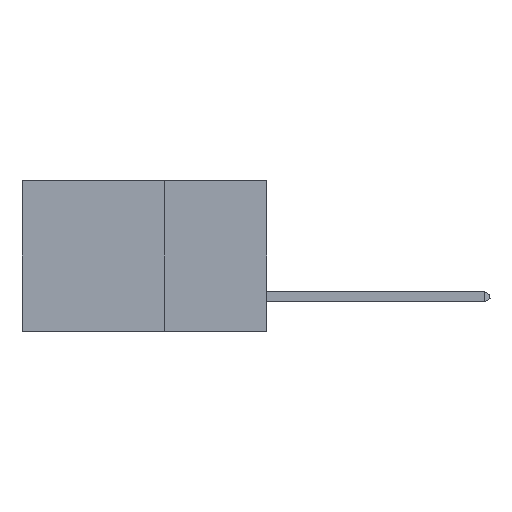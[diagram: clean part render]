
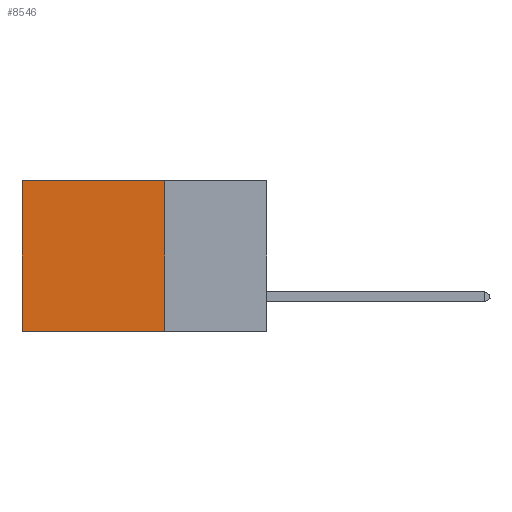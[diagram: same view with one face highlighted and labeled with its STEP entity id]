
A CAD part, left-side view. The second image highlights one B-rep face of the part: STEP entity #8546.
In plain terms, the highlighted planar face has unit normal (-1, 0, 0).
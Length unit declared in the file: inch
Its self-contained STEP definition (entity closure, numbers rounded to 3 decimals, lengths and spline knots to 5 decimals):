
#838 = DIRECTION ( 'NONE',  ( 0., 1., 0. ) ) ;
#1077 = CARTESIAN_POINT ( 'NONE',  ( 0.2875, 0.25, -0.37 ) ) ;
#1241 = EDGE_LOOP ( 'NONE', ( #8976, #8566, #4167, #13422 ) ) ;
#1479 = VECTOR ( 'NONE', #16630, 39.37008 ) ;
#1758 = VERTEX_POINT ( 'NONE', #14915 ) ;
#1759 = CARTESIAN_POINT ( 'NONE',  ( 0.2875, 0.6, 0. ) ) ;
#2491 = LINE ( 'NONE', #5364, #2725 ) ;
#2725 = VECTOR ( 'NONE', #15488, 39.37008 ) ;
#2835 = PLANE ( 'NONE',  #13558 ) ;
#3057 = VERTEX_POINT ( 'NONE', #8640 ) ;
#3827 = CARTESIAN_POINT ( 'NONE',  ( 0.2875, 0.25, -0.37 ) ) ;
#4167 = ORIENTED_EDGE ( 'NONE', *, *, #18535, .F. ) ;
#4817 = VERTEX_POINT ( 'NONE', #9337 ) ;
#5364 = CARTESIAN_POINT ( 'NONE',  ( 0.2875, 0.25, 0. ) ) ;
#5885 = EDGE_CURVE ( 'NONE', #10804, #3057, #6015, .T. ) ;
#6015 = LINE ( 'NONE', #3827, #12172 ) ;
#6638 = LINE ( 'NONE', #1759, #18186 ) ;
#7819 = EDGE_CURVE ( 'NONE', #4817, #3057, #6638, .T. ) ;
#8546 = ADVANCED_FACE ( 'NONE', ( #9804 ), #2835, .F. ) ;
#8566 = ORIENTED_EDGE ( 'NONE', *, *, #5885, .F. ) ;
#8640 = CARTESIAN_POINT ( 'NONE',  ( 0.2875, 0.6, -0.37 ) ) ;
#8976 = ORIENTED_EDGE ( 'NONE', *, *, #7819, .T. ) ;
#9337 = CARTESIAN_POINT ( 'NONE',  ( 0.2875, 0.6, 0. ) ) ;
#9804 = FACE_OUTER_BOUND ( 'NONE', #1241, .T. ) ;
#10077 = DIRECTION ( 'NONE',  ( 1., 0., 0. ) ) ;
#10343 = EDGE_CURVE ( 'NONE', #1758, #4817, #2491, .T. ) ;
#10804 = VERTEX_POINT ( 'NONE', #1077 ) ;
#11904 = DIRECTION ( 'NONE',  ( 0., 0., -1. ) ) ;
#12172 = VECTOR ( 'NONE', #838, 39.37008 ) ;
#12220 = CARTESIAN_POINT ( 'NONE',  ( 0.2875, 0.25, 0. ) ) ;
#12311 = LINE ( 'NONE', #12220, #1479 ) ;
#13422 = ORIENTED_EDGE ( 'NONE', *, *, #10343, .T. ) ;
#13558 = AXIS2_PLACEMENT_3D ( 'NONE', #14385, #10077, #14446 ) ;
#14385 = CARTESIAN_POINT ( 'NONE',  ( 0.2875, 0.25, 0. ) ) ;
#14446 = DIRECTION ( 'NONE',  ( 0., 0., -1. ) ) ;
#14915 = CARTESIAN_POINT ( 'NONE',  ( 0.2875, 0.25, 0. ) ) ;
#15488 = DIRECTION ( 'NONE',  ( 0., 1., 0. ) ) ;
#16630 = DIRECTION ( 'NONE',  ( 0., 0., -1. ) ) ;
#18186 = VECTOR ( 'NONE', #11904, 39.37008 ) ;
#18535 = EDGE_CURVE ( 'NONE', #1758, #10804, #12311, .T. ) ;
